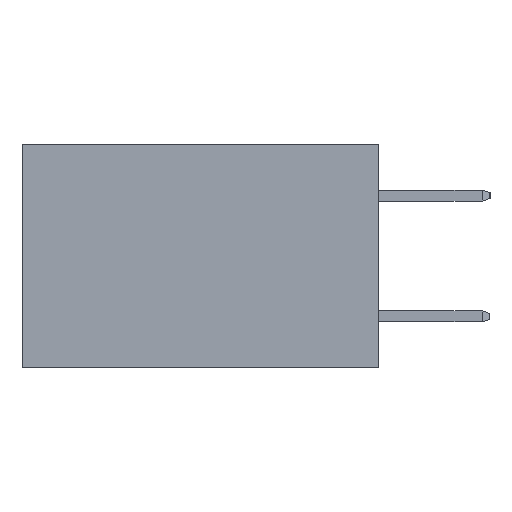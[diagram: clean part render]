
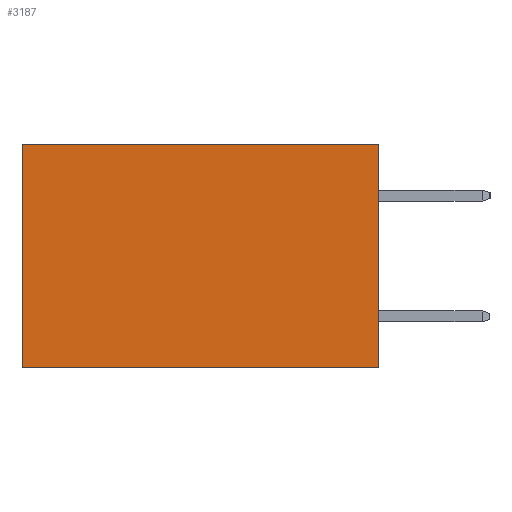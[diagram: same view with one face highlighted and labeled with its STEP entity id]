
A CAD part, left-side view. The second image highlights one B-rep face of the part: STEP entity #3187.
In plain terms, the highlighted planar face has unit normal (-1, 0, 0).
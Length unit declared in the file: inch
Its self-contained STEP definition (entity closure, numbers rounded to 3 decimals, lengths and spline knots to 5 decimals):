
#97 = DIRECTION ( 'NONE',  ( 0., 1., 0. ) ) ;
#978 = EDGE_CURVE ( 'NONE', #6412, #13510, #7033, .T. ) ;
#1156 = CARTESIAN_POINT ( 'NONE',  ( 0.277, 0., 0. ) ) ;
#1204 = EDGE_CURVE ( 'NONE', #13510, #4556, #3980, .T. ) ;
#1358 = CARTESIAN_POINT ( 'NONE',  ( 0.277, 0.59, 0. ) ) ;
#1760 = DIRECTION ( 'NONE',  ( 0., 0., -1. ) ) ;
#3187 = ADVANCED_FACE ( 'NONE', ( #12395 ), #8681, .F. ) ;
#3980 = LINE ( 'NONE', #12490, #12856 ) ;
#4556 = VERTEX_POINT ( 'NONE', #15396 ) ;
#5119 = CARTESIAN_POINT ( 'NONE',  ( 0.277, 0., -0.37 ) ) ;
#6412 = VERTEX_POINT ( 'NONE', #1156 ) ;
#6514 = ORIENTED_EDGE ( 'NONE', *, *, #12396, .F. ) ;
#6755 = CARTESIAN_POINT ( 'NONE',  ( 0.277, 0., 0. ) ) ;
#7033 = LINE ( 'NONE', #6755, #14780 ) ;
#7139 = CARTESIAN_POINT ( 'NONE',  ( 0.277, 0., -0.37 ) ) ;
#7387 = DIRECTION ( 'NONE',  ( 0., 0., -1. ) ) ;
#7390 = DIRECTION ( 'NONE',  ( 1., 0., 0. ) ) ;
#7699 = ORIENTED_EDGE ( 'NONE', *, *, #10066, .F. ) ;
#8188 = ORIENTED_EDGE ( 'NONE', *, *, #1204, .T. ) ;
#8437 = CARTESIAN_POINT ( 'NONE',  ( 0.277, 0., -0.37 ) ) ;
#8681 = PLANE ( 'NONE',  #14536 ) ;
#10060 = ORIENTED_EDGE ( 'NONE', *, *, #978, .T. ) ;
#10066 = EDGE_CURVE ( 'NONE', #12110, #4556, #10669, .T. ) ;
#10222 = EDGE_LOOP ( 'NONE', ( #8188, #7699, #6514, #10060 ) ) ;
#10669 = LINE ( 'NONE', #14418, #13706 ) ;
#10677 = VECTOR ( 'NONE', #15333, 39.37008 ) ;
#12110 = VERTEX_POINT ( 'NONE', #7139 ) ;
#12149 = DIRECTION ( 'NONE',  ( 0., 1., 0. ) ) ;
#12395 = FACE_OUTER_BOUND ( 'NONE', #10222, .T. ) ;
#12396 = EDGE_CURVE ( 'NONE', #6412, #12110, #13719, .T. ) ;
#12490 = CARTESIAN_POINT ( 'NONE',  ( 0.277, 0.59, -0.37 ) ) ;
#12856 = VECTOR ( 'NONE', #1760, 39.37008 ) ;
#13510 = VERTEX_POINT ( 'NONE', #1358 ) ;
#13706 = VECTOR ( 'NONE', #12149, 39.37008 ) ;
#13719 = LINE ( 'NONE', #5119, #10677 ) ;
#14418 = CARTESIAN_POINT ( 'NONE',  ( 0.277, 0., -0.37 ) ) ;
#14536 = AXIS2_PLACEMENT_3D ( 'NONE', #8437, #7390, #7387 ) ;
#14780 = VECTOR ( 'NONE', #97, 39.37008 ) ;
#15333 = DIRECTION ( 'NONE',  ( 0., 0., -1. ) ) ;
#15396 = CARTESIAN_POINT ( 'NONE',  ( 0.277, 0.59, -0.37 ) ) ;
